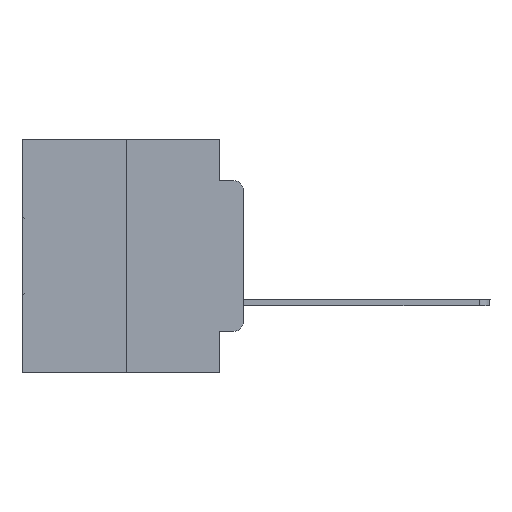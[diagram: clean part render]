
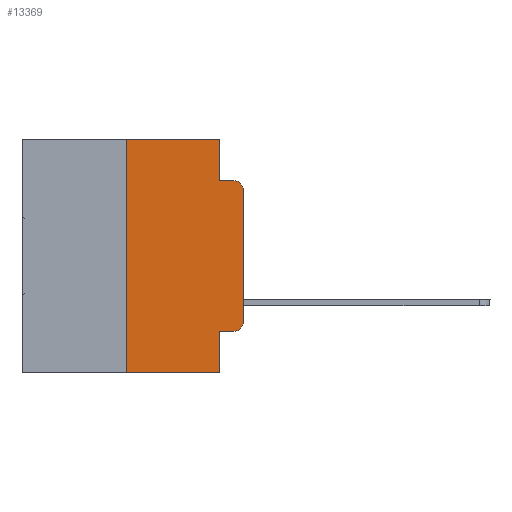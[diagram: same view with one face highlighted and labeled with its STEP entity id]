
A CAD part, left-side view. The second image highlights one B-rep face of the part: STEP entity #13369.
In plain terms, the highlighted planar face has unit normal (-1, 0, 0).
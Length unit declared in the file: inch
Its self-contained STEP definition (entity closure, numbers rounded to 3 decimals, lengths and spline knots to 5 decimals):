
#718 = ORIENTED_EDGE ( 'NONE', *, *, #17409, .F. ) ;
#854 = EDGE_LOOP ( 'NONE', ( #13447, #17634, #19124, #718, #6612, #9542, #16503, #7210, #23116, #22156 ) ) ;
#1834 = LINE ( 'NONE', #18973, #4184 ) ;
#1839 = LINE ( 'NONE', #13979, #29237 ) ;
#2062 = VERTEX_POINT ( 'NONE', #23217 ) ;
#2183 = CARTESIAN_POINT ( 'NONE',  ( 0., 0.051, 0. ) ) ;
#2200 = CARTESIAN_POINT ( 'NONE',  ( 0., 0.051, -0.0885 ) ) ;
#2708 = DIRECTION ( 'NONE',  ( -1., 0., 0. ) ) ;
#3803 = EDGE_CURVE ( 'NONE', #16226, #20578, #18724, .T. ) ;
#4184 = VECTOR ( 'NONE', #21895, 39.37008 ) ;
#5142 = EDGE_CURVE ( 'NONE', #16733, #2062, #12876, .T. ) ;
#5394 = CARTESIAN_POINT ( 'NONE',  ( 0., 0.051, -0.4115 ) ) ;
#6242 = CARTESIAN_POINT ( 'NONE',  ( 0., 0.02, -0.4115 ) ) ;
#6612 = ORIENTED_EDGE ( 'NONE', *, *, #3803, .F. ) ;
#6873 = EDGE_CURVE ( 'NONE', #12047, #10162, #1839, .T. ) ;
#7195 = FACE_OUTER_BOUND ( 'NONE', #854, .T. ) ;
#7210 = ORIENTED_EDGE ( 'NONE', *, *, #8067, .F. ) ;
#7516 = DIRECTION ( 'NONE',  ( 1., 0., 0. ) ) ;
#8067 = EDGE_CURVE ( 'NONE', #29664, #10162, #20951, .T. ) ;
#8995 = LINE ( 'NONE', #2183, #22418 ) ;
#9272 = EDGE_CURVE ( 'NONE', #2062, #11990, #23673, .T. ) ;
#9474 = CARTESIAN_POINT ( 'NONE',  ( 0., 0.473, 0. ) ) ;
#9495 = VECTOR ( 'NONE', #21805, 39.37008 ) ;
#9542 = ORIENTED_EDGE ( 'NONE', *, *, #27712, .F. ) ;
#10162 = VERTEX_POINT ( 'NONE', #24775 ) ;
#11285 = EDGE_CURVE ( 'NONE', #18603, #16733, #16533, .T. ) ;
#11990 = VERTEX_POINT ( 'NONE', #20811 ) ;
#12047 = VERTEX_POINT ( 'NONE', #15946 ) ;
#12143 = VECTOR ( 'NONE', #15464, 39.37008 ) ;
#12633 = CARTESIAN_POINT ( 'NONE',  ( 0., 0.25, 0. ) ) ;
#12876 = LINE ( 'NONE', #20324, #12143 ) ;
#13369 = ADVANCED_FACE ( 'NONE', ( #7195 ), #29234, .F. ) ;
#13447 = ORIENTED_EDGE ( 'NONE', *, *, #5142, .T. ) ;
#13534 = EDGE_CURVE ( 'NONE', #29664, #18603, #27597, .T. ) ;
#13979 = CARTESIAN_POINT ( 'NONE',  ( 0., 0.473, -0.5 ) ) ;
#14280 = DIRECTION ( 'NONE',  ( 0., 0., -1. ) ) ;
#14477 = DIRECTION ( 'NONE',  ( 0., 0., -1. ) ) ;
#15021 = VECTOR ( 'NONE', #27436, 39.37008 ) ;
#15464 = DIRECTION ( 'NONE',  ( 0., 0., 1. ) ) ;
#15605 = DIRECTION ( 'NONE',  ( 0., 0., -1. ) ) ;
#15946 = CARTESIAN_POINT ( 'NONE',  ( 0., 0.25, -0.5 ) ) ;
#16095 = DIRECTION ( 'NONE',  ( 0., 0., -1. ) ) ;
#16226 = VERTEX_POINT ( 'NONE', #12633 ) ;
#16503 = ORIENTED_EDGE ( 'NONE', *, *, #6873, .T. ) ;
#16533 = CIRCLE ( 'NONE', #26362, 0.02 ) ;
#16733 = VERTEX_POINT ( 'NONE', #25229 ) ;
#16779 = CARTESIAN_POINT ( 'NONE',  ( 0., 0.473, 0. ) ) ;
#16881 = DIRECTION ( 'NONE',  ( 0., -1., 0. ) ) ;
#17409 = EDGE_CURVE ( 'NONE', #20578, #17881, #8995, .T. ) ;
#17634 = ORIENTED_EDGE ( 'NONE', *, *, #9272, .T. ) ;
#17881 = VERTEX_POINT ( 'NONE', #21254 ) ;
#18033 = CARTESIAN_POINT ( 'NONE',  ( 0., 0.02, -0.1085 ) ) ;
#18486 = AXIS2_PLACEMENT_3D ( 'NONE', #18033, #2708, #15605 ) ;
#18603 = VERTEX_POINT ( 'NONE', #6242 ) ;
#18724 = LINE ( 'NONE', #16779, #9495 ) ;
#18973 = CARTESIAN_POINT ( 'NONE',  ( 0., 0.25, 0. ) ) ;
#19124 = ORIENTED_EDGE ( 'NONE', *, *, #25948, .F. ) ;
#19647 = DIRECTION ( 'NONE',  ( 0., 0., -1. ) ) ;
#20324 = CARTESIAN_POINT ( 'NONE',  ( 0., 0., 0. ) ) ;
#20578 = VERTEX_POINT ( 'NONE', #29474 ) ;
#20788 = CARTESIAN_POINT ( 'NONE',  ( 0., 0.051, 0. ) ) ;
#20811 = CARTESIAN_POINT ( 'NONE',  ( 0., 0.02, -0.0885 ) ) ;
#20951 = LINE ( 'NONE', #20788, #24147 ) ;
#21254 = CARTESIAN_POINT ( 'NONE',  ( 0., 0.051, -0.0885 ) ) ;
#21805 = DIRECTION ( 'NONE',  ( 0., -1., 0. ) ) ;
#21895 = DIRECTION ( 'NONE',  ( 0., 0., 1. ) ) ;
#22102 = DIRECTION ( 'NONE',  ( 0., -1., 0. ) ) ;
#22156 = ORIENTED_EDGE ( 'NONE', *, *, #11285, .T. ) ;
#22321 = CARTESIAN_POINT ( 'NONE',  ( 0., 0.02, -0.3915 ) ) ;
#22418 = VECTOR ( 'NONE', #14477, 39.37008 ) ;
#23116 = ORIENTED_EDGE ( 'NONE', *, *, #13534, .T. ) ;
#23217 = CARTESIAN_POINT ( 'NONE',  ( 0., 0., -0.1085 ) ) ;
#23673 = CIRCLE ( 'NONE', #18486, 0.02 ) ;
#24147 = VECTOR ( 'NONE', #16095, 39.37008 ) ;
#24775 = CARTESIAN_POINT ( 'NONE',  ( 0., 0.051, -0.5 ) ) ;
#25229 = CARTESIAN_POINT ( 'NONE',  ( 0., 0., -0.3915 ) ) ;
#25948 = EDGE_CURVE ( 'NONE', #17881, #11990, #26972, .T. ) ;
#26362 = AXIS2_PLACEMENT_3D ( 'NONE', #22321, #26591, #14280 ) ;
#26591 = DIRECTION ( 'NONE',  ( -1., 0., 0. ) ) ;
#26972 = LINE ( 'NONE', #2200, #28409 ) ;
#27436 = DIRECTION ( 'NONE',  ( 0., -1., 0. ) ) ;
#27597 = LINE ( 'NONE', #5394, #15021 ) ;
#27712 = EDGE_CURVE ( 'NONE', #12047, #16226, #1834, .T. ) ;
#28174 = CARTESIAN_POINT ( 'NONE',  ( 0., 0.051, -0.4115 ) ) ;
#28409 = VECTOR ( 'NONE', #22102, 39.37008 ) ;
#29234 = PLANE ( 'NONE',  #31579 ) ;
#29237 = VECTOR ( 'NONE', #16881, 39.37008 ) ;
#29474 = CARTESIAN_POINT ( 'NONE',  ( 0., 0.051, 0. ) ) ;
#29664 = VERTEX_POINT ( 'NONE', #28174 ) ;
#31579 = AXIS2_PLACEMENT_3D ( 'NONE', #9474, #7516, #19647 ) ;
